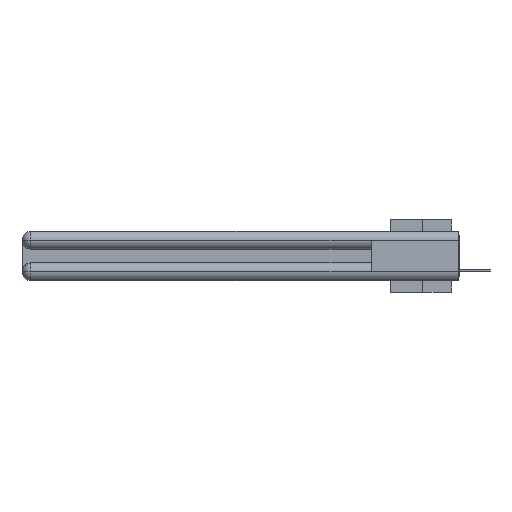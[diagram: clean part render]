
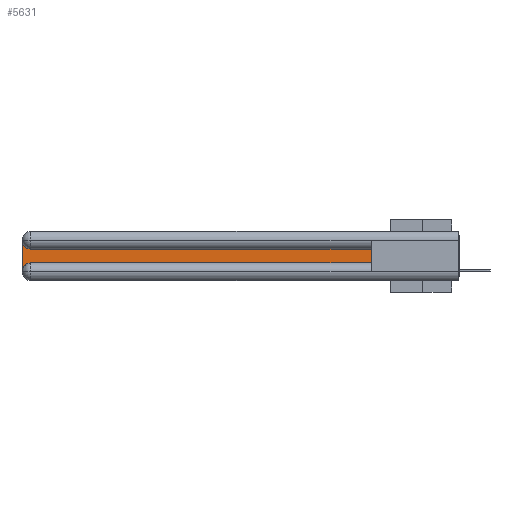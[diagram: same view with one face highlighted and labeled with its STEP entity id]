
A CAD part, left-side view. The second image highlights one B-rep face of the part: STEP entity #5631.
In plain terms, the highlighted planar face has unit normal (-1, 0, 0).
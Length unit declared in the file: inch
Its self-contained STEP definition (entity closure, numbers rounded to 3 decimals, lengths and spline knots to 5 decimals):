
#2 = AXIS2_PLACEMENT_3D ( 'NONE', #27569, #23026, #2408 ) ;
#1512 = VECTOR ( 'NONE', #23245, 39.37008 ) ;
#1784 = EDGE_LOOP ( 'NONE', ( #21835, #21533, #7828, #14716, #17840, #27212 ) ) ;
#2408 = DIRECTION ( 'NONE',  ( 0., 0., -1. ) ) ;
#2932 = DIRECTION ( 'NONE',  ( 1., 0., 0. ) ) ;
#3318 = CARTESIAN_POINT ( 'NONE',  ( 0.075, 0.6, -0.2175 ) ) ;
#5181 = AXIS2_PLACEMENT_3D ( 'NONE', #11840, #18769, #9326 ) ;
#5631 = ADVANCED_FACE ( 'NONE', ( #14186 ), #20755, .F. ) ;
#6050 = VERTEX_POINT ( 'NONE', #29280 ) ;
#6337 = EDGE_CURVE ( 'NONE', #8173, #15716, #13470, .T. ) ;
#6818 = VECTOR ( 'NONE', #22464, 39.37008 ) ;
#7828 = ORIENTED_EDGE ( 'NONE', *, *, #28295, .T. ) ;
#8173 = VERTEX_POINT ( 'NONE', #14849 ) ;
#8248 = LINE ( 'NONE', #24385, #6818 ) ;
#8971 = DIRECTION ( 'NONE',  ( 0., -1., 0. ) ) ;
#9326 = DIRECTION ( 'NONE',  ( 0., 0., -1. ) ) ;
#9910 = CARTESIAN_POINT ( 'NONE',  ( 0.075, 2.94, -0.0625 ) ) ;
#10669 = LINE ( 'NONE', #11456, #14647 ) ;
#11456 = CARTESIAN_POINT ( 'NONE',  ( 0.075, 0.6, -0.1225 ) ) ;
#11630 = CARTESIAN_POINT ( 'NONE',  ( 0.075, 0.6, -0.2175 ) ) ;
#11840 = CARTESIAN_POINT ( 'NONE',  ( 0.075, 3., -0.1225 ) ) ;
#13185 = CIRCLE ( 'NONE', #2, 0.06 ) ;
#13451 = EDGE_CURVE ( 'NONE', #25904, #6050, #18821, .T. ) ;
#13470 = CIRCLE ( 'NONE', #22516, 0.06 ) ;
#14186 = FACE_OUTER_BOUND ( 'NONE', #1784, .T. ) ;
#14647 = VECTOR ( 'NONE', #25482, 39.37008 ) ;
#14716 = ORIENTED_EDGE ( 'NONE', *, *, #18562, .T. ) ;
#14849 = CARTESIAN_POINT ( 'NONE',  ( 0.075, 2.94, -0.1225 ) ) ;
#15716 = VERTEX_POINT ( 'NONE', #17534 ) ;
#15915 = EDGE_CURVE ( 'NONE', #27735, #25904, #18344, .T. ) ;
#17419 = CARTESIAN_POINT ( 'NONE',  ( 0.075, 2.94, -0.2175 ) ) ;
#17534 = CARTESIAN_POINT ( 'NONE',  ( 0.075, 3., -0.0625 ) ) ;
#17636 = VERTEX_POINT ( 'NONE', #26764 ) ;
#17840 = ORIENTED_EDGE ( 'NONE', *, *, #15915, .T. ) ;
#18344 = LINE ( 'NONE', #25032, #24421 ) ;
#18562 = EDGE_CURVE ( 'NONE', #17636, #27735, #13185, .T. ) ;
#18769 = DIRECTION ( 'NONE',  ( 1., 0., 0. ) ) ;
#18821 = LINE ( 'NONE', #11630, #1512 ) ;
#19031 = DIRECTION ( 'NONE',  ( 0., 0., -1. ) ) ;
#20755 = PLANE ( 'NONE',  #5181 ) ;
#21533 = ORIENTED_EDGE ( 'NONE', *, *, #6337, .T. ) ;
#21835 = ORIENTED_EDGE ( 'NONE', *, *, #23878, .T. ) ;
#22464 = DIRECTION ( 'NONE',  ( 0., 0., -1. ) ) ;
#22516 = AXIS2_PLACEMENT_3D ( 'NONE', #9910, #2932, #19031 ) ;
#23026 = DIRECTION ( 'NONE',  ( 1., 0., 0. ) ) ;
#23245 = DIRECTION ( 'NONE',  ( 0., 0., 1. ) ) ;
#23878 = EDGE_CURVE ( 'NONE', #6050, #8173, #10669, .T. ) ;
#24385 = CARTESIAN_POINT ( 'NONE',  ( 0.075, 3., -0.2175 ) ) ;
#24421 = VECTOR ( 'NONE', #8971, 39.37008 ) ;
#25032 = CARTESIAN_POINT ( 'NONE',  ( 0.075, 0.6, -0.2175 ) ) ;
#25482 = DIRECTION ( 'NONE',  ( 0., 1., 0. ) ) ;
#25904 = VERTEX_POINT ( 'NONE', #3318 ) ;
#26764 = CARTESIAN_POINT ( 'NONE',  ( 0.075, 3., -0.2775 ) ) ;
#27212 = ORIENTED_EDGE ( 'NONE', *, *, #13451, .T. ) ;
#27569 = CARTESIAN_POINT ( 'NONE',  ( 0.075, 2.94, -0.2775 ) ) ;
#27735 = VERTEX_POINT ( 'NONE', #17419 ) ;
#28295 = EDGE_CURVE ( 'NONE', #15716, #17636, #8248, .T. ) ;
#29280 = CARTESIAN_POINT ( 'NONE',  ( 0.075, 0.6, -0.1225 ) ) ;
